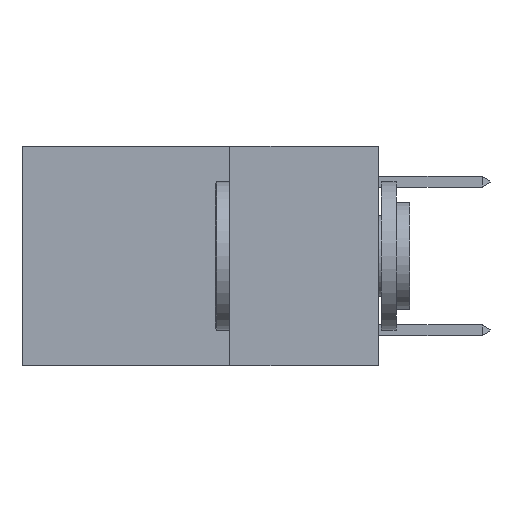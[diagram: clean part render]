
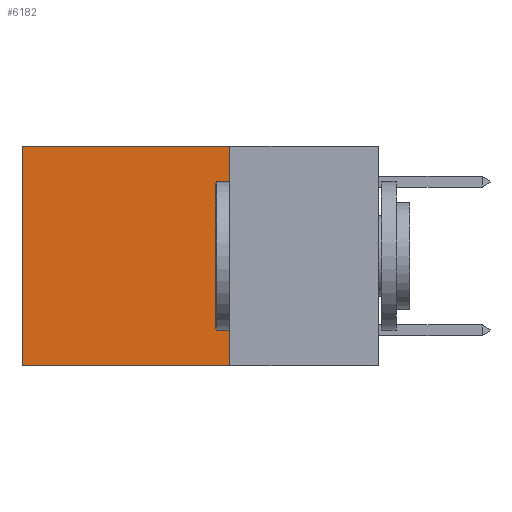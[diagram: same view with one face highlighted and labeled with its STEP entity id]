
A CAD part, left-side view. The second image highlights one B-rep face of the part: STEP entity #6182.
In plain terms, the highlighted planar face has unit normal (-1, 0, 0).
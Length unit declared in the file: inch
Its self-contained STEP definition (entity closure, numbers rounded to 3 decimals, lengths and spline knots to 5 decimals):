
#70 = CARTESIAN_POINT ( 'NONE',  ( 0.2625, 0.6, 0. ) ) ;
#550 = CARTESIAN_POINT ( 'NONE',  ( 0.2625, 0.6, -0.37 ) ) ;
#630 = CARTESIAN_POINT ( 'NONE',  ( 0.2625, 0.25, 0. ) ) ;
#1167 = DIRECTION ( 'NONE',  ( 1., 0., 0. ) ) ;
#1431 = CARTESIAN_POINT ( 'NONE',  ( 0.2625, 0.25, 0. ) ) ;
#1548 = CARTESIAN_POINT ( 'NONE',  ( 0.2625, 0.6, 0. ) ) ;
#1660 = DIRECTION ( 'NONE',  ( 0., 1., 0. ) ) ;
#2088 = ORIENTED_EDGE ( 'NONE', *, *, #9976, .F. ) ;
#2509 = PLANE ( 'NONE',  #9941 ) ;
#2663 = DIRECTION ( 'NONE',  ( 0., 0., -1. ) ) ;
#3086 = VERTEX_POINT ( 'NONE', #7431 ) ;
#3401 = VECTOR ( 'NONE', #12468, 39.37008 ) ;
#4080 = VECTOR ( 'NONE', #10052, 39.37008 ) ;
#4283 = ORIENTED_EDGE ( 'NONE', *, *, #6368, .T. ) ;
#5123 = ORIENTED_EDGE ( 'NONE', *, *, #12228, .T. ) ;
#5404 = CARTESIAN_POINT ( 'NONE',  ( 0.2625, 0.25, 0. ) ) ;
#5741 = VECTOR ( 'NONE', #1660, 39.37008 ) ;
#6182 = ADVANCED_FACE ( 'NONE', ( #12027 ), #2509, .F. ) ;
#6368 = EDGE_CURVE ( 'NONE', #13891, #7539, #6649, .T. ) ;
#6649 = LINE ( 'NONE', #1548, #4080 ) ;
#7431 = CARTESIAN_POINT ( 'NONE',  ( 0.2625, 0.25, -0.37 ) ) ;
#7481 = CARTESIAN_POINT ( 'NONE',  ( 0.2625, 0.25, -0.37 ) ) ;
#7539 = VERTEX_POINT ( 'NONE', #550 ) ;
#7554 = LINE ( 'NONE', #7481, #9494 ) ;
#8169 = EDGE_LOOP ( 'NONE', ( #4283, #2088, #11397, #5123 ) ) ;
#9114 = LINE ( 'NONE', #630, #5741 ) ;
#9144 = LINE ( 'NONE', #5404, #3401 ) ;
#9494 = VECTOR ( 'NONE', #14774, 39.37008 ) ;
#9941 = AXIS2_PLACEMENT_3D ( 'NONE', #10906, #1167, #2663 ) ;
#9976 = EDGE_CURVE ( 'NONE', #3086, #7539, #7554, .T. ) ;
#10052 = DIRECTION ( 'NONE',  ( 0., 0., -1. ) ) ;
#10057 = EDGE_CURVE ( 'NONE', #10517, #3086, #9144, .T. ) ;
#10517 = VERTEX_POINT ( 'NONE', #1431 ) ;
#10906 = CARTESIAN_POINT ( 'NONE',  ( 0.2625, 0.25, 0. ) ) ;
#11397 = ORIENTED_EDGE ( 'NONE', *, *, #10057, .F. ) ;
#12027 = FACE_OUTER_BOUND ( 'NONE', #8169, .T. ) ;
#12228 = EDGE_CURVE ( 'NONE', #10517, #13891, #9114, .T. ) ;
#12468 = DIRECTION ( 'NONE',  ( 0., 0., -1. ) ) ;
#13891 = VERTEX_POINT ( 'NONE', #70 ) ;
#14774 = DIRECTION ( 'NONE',  ( 0., 1., 0. ) ) ;
